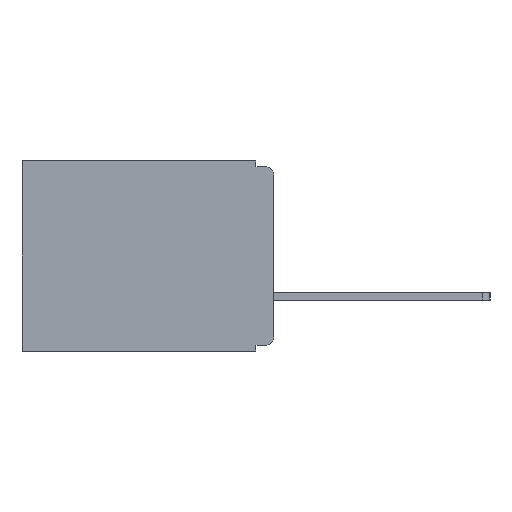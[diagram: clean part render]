
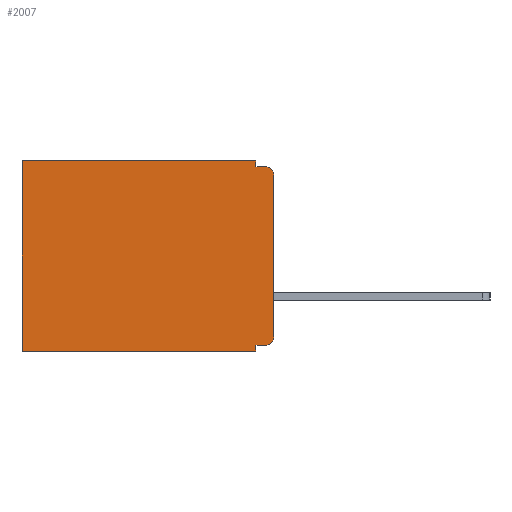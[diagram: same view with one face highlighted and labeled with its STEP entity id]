
A CAD part, left-side view. The second image highlights one B-rep face of the part: STEP entity #2007.
In plain terms, the highlighted planar face has unit normal (-1, 0, 0).
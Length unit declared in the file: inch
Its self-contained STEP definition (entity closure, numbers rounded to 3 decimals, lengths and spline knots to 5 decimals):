
#432 = CARTESIAN_POINT ( 'NONE',  ( 0.3, 0.437, -0.33 ) ) ;
#835 = LINE ( 'NONE', #26661, #13550 ) ;
#858 = CARTESIAN_POINT ( 'NONE',  ( 0.3, 0.437, -0.33 ) ) ;
#1063 = AXIS2_PLACEMENT_3D ( 'NONE', #20945, #20911, #20783 ) ;
#1757 = DIRECTION ( 'NONE',  ( 0., 0., -1. ) ) ;
#2007 = ADVANCED_FACE ( 'NONE', ( #21202 ), #12667, .F. ) ;
#2020 = VERTEX_POINT ( 'NONE', #432 ) ;
#2535 = EDGE_CURVE ( 'NONE', #14769, #2600, #25440, .T. ) ;
#2600 = VERTEX_POINT ( 'NONE', #23161 ) ;
#3704 = ORIENTED_EDGE ( 'NONE', *, *, #23872, .T. ) ;
#3772 = CARTESIAN_POINT ( 'NONE',  ( 0.3, 0., -0.025 ) ) ;
#3799 = DIRECTION ( 'NONE',  ( 0., 0., -1. ) ) ;
#5446 = LINE ( 'NONE', #25615, #31219 ) ;
#5639 = VERTEX_POINT ( 'NONE', #21976 ) ;
#5775 = ORIENTED_EDGE ( 'NONE', *, *, #7161, .T. ) ;
#6248 = VECTOR ( 'NONE', #31935, 39.37008 ) ;
#6291 = CARTESIAN_POINT ( 'NONE',  ( 0.3, 0., -0.305 ) ) ;
#6461 = VERTEX_POINT ( 'NONE', #6291 ) ;
#7126 = EDGE_CURVE ( 'NONE', #20478, #6461, #31333, .T. ) ;
#7161 = EDGE_CURVE ( 'NONE', #24089, #2020, #10728, .T. ) ;
#7533 = ORIENTED_EDGE ( 'NONE', *, *, #2535, .F. ) ;
#7994 = EDGE_CURVE ( 'NONE', #25051, #9024, #18093, .T. ) ;
#8127 = DIRECTION ( 'NONE',  ( 0., 1., 0. ) ) ;
#8853 = EDGE_CURVE ( 'NONE', #2600, #2020, #5446, .T. ) ;
#9024 = VERTEX_POINT ( 'NONE', #11313 ) ;
#9896 = ORIENTED_EDGE ( 'NONE', *, *, #17910, .F. ) ;
#10300 = DIRECTION ( 'NONE',  ( 0., 1., 0. ) ) ;
#10728 = LINE ( 'NONE', #858, #17370 ) ;
#11313 = CARTESIAN_POINT ( 'NONE',  ( 0.3, 0.015, -0.01 ) ) ;
#12667 = PLANE ( 'NONE',  #13517 ) ;
#12791 = AXIS2_PLACEMENT_3D ( 'NONE', #29778, #14893, #32198 ) ;
#12801 = LINE ( 'NONE', #17845, #31810 ) ;
#13415 = ORIENTED_EDGE ( 'NONE', *, *, #7994, .T. ) ;
#13517 = AXIS2_PLACEMENT_3D ( 'NONE', #21205, #15394, #22371 ) ;
#13550 = VECTOR ( 'NONE', #19269, 39.37008 ) ;
#14769 = VERTEX_POINT ( 'NONE', #17635 ) ;
#14893 = DIRECTION ( 'NONE',  ( -1., 0., 0. ) ) ;
#15394 = DIRECTION ( 'NONE',  ( 1., 0., 0. ) ) ;
#16086 = DIRECTION ( 'NONE',  ( 0., 1., 0. ) ) ;
#16304 = EDGE_LOOP ( 'NONE', ( #29795, #13415, #9896, #18129, #3704, #5775, #17162, #7533, #23261, #24260 ) ) ;
#16447 = EDGE_CURVE ( 'NONE', #17509, #5639, #28503, .T. ) ;
#17072 = VECTOR ( 'NONE', #27692, 39.37008 ) ;
#17162 = ORIENTED_EDGE ( 'NONE', *, *, #8853, .F. ) ;
#17245 = LINE ( 'NONE', #30936, #30434 ) ;
#17370 = VECTOR ( 'NONE', #3799, 39.37008 ) ;
#17509 = VERTEX_POINT ( 'NONE', #31003 ) ;
#17635 = CARTESIAN_POINT ( 'NONE',  ( 0.3, 0.031, -0.32 ) ) ;
#17756 = CARTESIAN_POINT ( 'NONE',  ( 0.3, 0., -0.01 ) ) ;
#17845 = CARTESIAN_POINT ( 'NONE',  ( 0.3, 0., -0.32 ) ) ;
#17910 = EDGE_CURVE ( 'NONE', #5639, #9024, #22133, .T. ) ;
#18093 = CIRCLE ( 'NONE', #12791, 0.015 ) ;
#18129 = ORIENTED_EDGE ( 'NONE', *, *, #16447, .F. ) ;
#19269 = DIRECTION ( 'NONE',  ( 0., 0., -1. ) ) ;
#20478 = VERTEX_POINT ( 'NONE', #22175 ) ;
#20783 = DIRECTION ( 'NONE',  ( 0., 0., -1. ) ) ;
#20911 = DIRECTION ( 'NONE',  ( -1., 0., 0. ) ) ;
#20945 = CARTESIAN_POINT ( 'NONE',  ( 0.3, 0.015, -0.305 ) ) ;
#21202 = FACE_OUTER_BOUND ( 'NONE', #16304, .T. ) ;
#21205 = CARTESIAN_POINT ( 'NONE',  ( 0.3, 0., -0.33 ) ) ;
#21840 = CARTESIAN_POINT ( 'NONE',  ( 0.3, 0.437, 0. ) ) ;
#21976 = CARTESIAN_POINT ( 'NONE',  ( 0.3, 0.031, -0.01 ) ) ;
#22133 = LINE ( 'NONE', #17756, #17072 ) ;
#22175 = CARTESIAN_POINT ( 'NONE',  ( 0.3, 0.015, -0.32 ) ) ;
#22371 = DIRECTION ( 'NONE',  ( 0., 0., -1. ) ) ;
#22642 = VECTOR ( 'NONE', #1757, 39.37008 ) ;
#23161 = CARTESIAN_POINT ( 'NONE',  ( 0.3, 0.031, -0.33 ) ) ;
#23261 = ORIENTED_EDGE ( 'NONE', *, *, #26606, .F. ) ;
#23872 = EDGE_CURVE ( 'NONE', #17509, #24089, #17245, .T. ) ;
#24089 = VERTEX_POINT ( 'NONE', #21840 ) ;
#24260 = ORIENTED_EDGE ( 'NONE', *, *, #7126, .T. ) ;
#25051 = VERTEX_POINT ( 'NONE', #3772 ) ;
#25440 = LINE ( 'NONE', #27533, #6248 ) ;
#25615 = CARTESIAN_POINT ( 'NONE',  ( 0.3, 0., -0.33 ) ) ;
#26606 = EDGE_CURVE ( 'NONE', #20478, #14769, #12801, .T. ) ;
#26661 = CARTESIAN_POINT ( 'NONE',  ( 0.3, 0., -0.33 ) ) ;
#26902 = CARTESIAN_POINT ( 'NONE',  ( 0.3, 0.031, 0. ) ) ;
#26990 = EDGE_CURVE ( 'NONE', #25051, #6461, #835, .T. ) ;
#27533 = CARTESIAN_POINT ( 'NONE',  ( 0.3, 0.031, -0.33 ) ) ;
#27692 = DIRECTION ( 'NONE',  ( 0., -1., 0. ) ) ;
#28503 = LINE ( 'NONE', #26902, #22642 ) ;
#29778 = CARTESIAN_POINT ( 'NONE',  ( 0.3, 0.015, -0.025 ) ) ;
#29795 = ORIENTED_EDGE ( 'NONE', *, *, #26990, .F. ) ;
#30434 = VECTOR ( 'NONE', #16086, 39.37008 ) ;
#30936 = CARTESIAN_POINT ( 'NONE',  ( 0.3, 0., 0. ) ) ;
#31003 = CARTESIAN_POINT ( 'NONE',  ( 0.3, 0.031, 0. ) ) ;
#31219 = VECTOR ( 'NONE', #8127, 39.37008 ) ;
#31333 = CIRCLE ( 'NONE', #1063, 0.015 ) ;
#31810 = VECTOR ( 'NONE', #10300, 39.37008 ) ;
#31935 = DIRECTION ( 'NONE',  ( 0., 0., -1. ) ) ;
#32198 = DIRECTION ( 'NONE',  ( 0., 0., -1. ) ) ;
